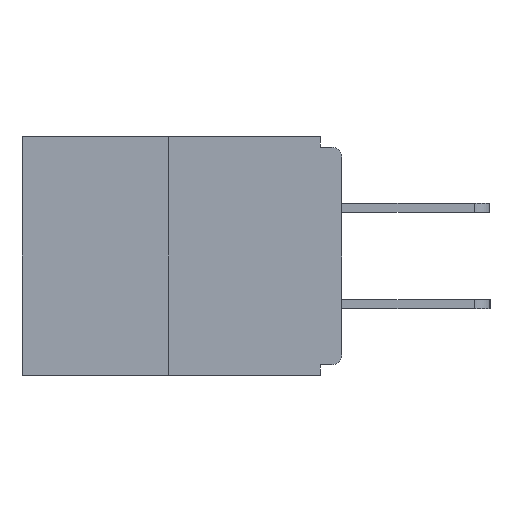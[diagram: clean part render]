
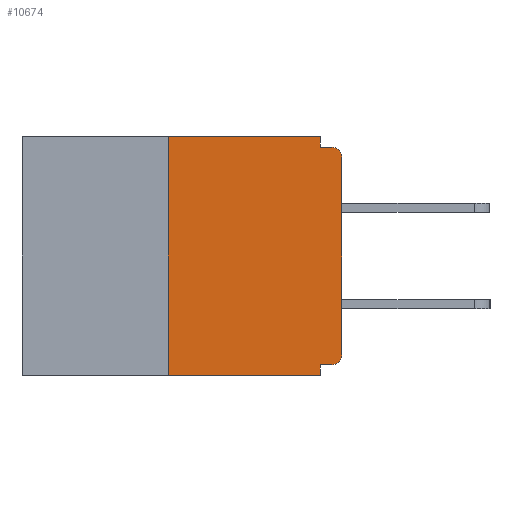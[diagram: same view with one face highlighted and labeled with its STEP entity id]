
A CAD part, left-side view. The second image highlights one B-rep face of the part: STEP entity #10674.
In plain terms, the highlighted planar face has unit normal (-1, 0, 0).
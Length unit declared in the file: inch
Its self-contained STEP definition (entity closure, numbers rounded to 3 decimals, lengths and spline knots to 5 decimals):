
#188 = LINE ( 'NONE', #837, #4559 ) ;
#520 = CARTESIAN_POINT ( 'NONE',  ( 0., 0.015, -0.03 ) ) ;
#718 = VECTOR ( 'NONE', #12293, 39.37008 ) ;
#837 = CARTESIAN_POINT ( 'NONE',  ( 0., 0., 0. ) ) ;
#1148 = VECTOR ( 'NONE', #7098, 39.37008 ) ;
#1250 = DIRECTION ( 'NONE',  ( 1., 0., 0. ) ) ;
#1312 = ORIENTED_EDGE ( 'NONE', *, *, #8876, .T. ) ;
#1439 = EDGE_LOOP ( 'NONE', ( #7261, #9956, #1312, #9376, #16176, #23420, #23938, #1974, #8960, #11372 ) ) ;
#1484 = CARTESIAN_POINT ( 'NONE',  ( 0., 0.031, -0.328 ) ) ;
#1597 = DIRECTION ( 'NONE',  ( 0., 0., 1. ) ) ;
#1974 = ORIENTED_EDGE ( 'NONE', *, *, #13596, .T. ) ;
#2115 = CARTESIAN_POINT ( 'NONE',  ( 0., 0., -0.313 ) ) ;
#2411 = LINE ( 'NONE', #10865, #6528 ) ;
#2457 = FACE_OUTER_BOUND ( 'NONE', #1439, .T. ) ;
#2822 = CARTESIAN_POINT ( 'NONE',  ( 0., 0., -0.015 ) ) ;
#3565 = EDGE_CURVE ( 'NONE', #16585, #7551, #13397, .T. ) ;
#3572 = CARTESIAN_POINT ( 'NONE',  ( 0., 0.46, -0.343 ) ) ;
#3648 = AXIS2_PLACEMENT_3D ( 'NONE', #520, #9982, #11940 ) ;
#4559 = VECTOR ( 'NONE', #19472, 39.37008 ) ;
#4700 = CARTESIAN_POINT ( 'NONE',  ( 0., 0.031, -0.015 ) ) ;
#4803 = CARTESIAN_POINT ( 'NONE',  ( 0., 0.46, 0. ) ) ;
#4838 = CARTESIAN_POINT ( 'NONE',  ( 0., 0.031, 0. ) ) ;
#5561 = LINE ( 'NONE', #3572, #15198 ) ;
#6234 = EDGE_CURVE ( 'NONE', #11658, #16585, #9492, .T. ) ;
#6528 = VECTOR ( 'NONE', #12492, 39.37008 ) ;
#7098 = DIRECTION ( 'NONE',  ( 0., -1., 0. ) ) ;
#7261 = ORIENTED_EDGE ( 'NONE', *, *, #6234, .F. ) ;
#7366 = DIRECTION ( 'NONE',  ( 0., -1., 0. ) ) ;
#7526 = CARTESIAN_POINT ( 'NONE',  ( 0., 0.25, 0. ) ) ;
#7551 = VERTEX_POINT ( 'NONE', #4700 ) ;
#7869 = VECTOR ( 'NONE', #9133, 39.37008 ) ;
#7979 = CARTESIAN_POINT ( 'NONE',  ( 0., 0.015, -0.313 ) ) ;
#8876 = EDGE_CURVE ( 'NONE', #20197, #20510, #5561, .T. ) ;
#8960 = ORIENTED_EDGE ( 'NONE', *, *, #22233, .F. ) ;
#9133 = DIRECTION ( 'NONE',  ( 0., 0., -1. ) ) ;
#9191 = CIRCLE ( 'NONE', #18291, 0.015 ) ;
#9376 = ORIENTED_EDGE ( 'NONE', *, *, #13749, .F. ) ;
#9492 = LINE ( 'NONE', #4803, #718 ) ;
#9520 = CARTESIAN_POINT ( 'NONE',  ( 0., 0.031, -0.343 ) ) ;
#9956 = ORIENTED_EDGE ( 'NONE', *, *, #10881, .F. ) ;
#9982 = DIRECTION ( 'NONE',  ( -1., 0., 0. ) ) ;
#10186 = CARTESIAN_POINT ( 'NONE',  ( 0., 0.015, -0.015 ) ) ;
#10621 = EDGE_CURVE ( 'NONE', #16329, #19788, #9191, .T. ) ;
#10674 = ADVANCED_FACE ( 'NONE', ( #2457 ), #16040, .F. ) ;
#10833 = CARTESIAN_POINT ( 'NONE',  ( 0., 0.25, -0.343 ) ) ;
#10856 = CARTESIAN_POINT ( 'NONE',  ( 0., 0.031, -0.343 ) ) ;
#10865 = CARTESIAN_POINT ( 'NONE',  ( 0., 0., -0.328 ) ) ;
#10881 = EDGE_CURVE ( 'NONE', #20197, #11658, #22971, .T. ) ;
#11372 = ORIENTED_EDGE ( 'NONE', *, *, #3565, .F. ) ;
#11658 = VERTEX_POINT ( 'NONE', #7526 ) ;
#11940 = DIRECTION ( 'NONE',  ( 0., 0., -1. ) ) ;
#12293 = DIRECTION ( 'NONE',  ( 0., -1., 0. ) ) ;
#12492 = DIRECTION ( 'NONE',  ( 0., 1., 0. ) ) ;
#12818 = VERTEX_POINT ( 'NONE', #10186 ) ;
#13397 = LINE ( 'NONE', #21056, #21026 ) ;
#13596 = EDGE_CURVE ( 'NONE', #20984, #12818, #18655, .T. ) ;
#13749 = EDGE_CURVE ( 'NONE', #21446, #20510, #22820, .T. ) ;
#14122 = VECTOR ( 'NONE', #1597, 39.37008 ) ;
#15198 = VECTOR ( 'NONE', #7366, 39.37008 ) ;
#16040 = PLANE ( 'NONE',  #16719 ) ;
#16176 = ORIENTED_EDGE ( 'NONE', *, *, #16833, .F. ) ;
#16329 = VERTEX_POINT ( 'NONE', #24001 ) ;
#16585 = VERTEX_POINT ( 'NONE', #4838 ) ;
#16719 = AXIS2_PLACEMENT_3D ( 'NONE', #23608, #1250, #19960 ) ;
#16833 = EDGE_CURVE ( 'NONE', #16329, #21446, #2411, .T. ) ;
#18291 = AXIS2_PLACEMENT_3D ( 'NONE', #7979, #21282, #21048 ) ;
#18655 = CIRCLE ( 'NONE', #3648, 0.015 ) ;
#19472 = DIRECTION ( 'NONE',  ( 0., 0., 1. ) ) ;
#19788 = VERTEX_POINT ( 'NONE', #2115 ) ;
#19960 = DIRECTION ( 'NONE',  ( 0., 0., -1. ) ) ;
#20197 = VERTEX_POINT ( 'NONE', #10833 ) ;
#20510 = VERTEX_POINT ( 'NONE', #9520 ) ;
#20531 = CARTESIAN_POINT ( 'NONE',  ( 0., 0., -0.03 ) ) ;
#20546 = EDGE_CURVE ( 'NONE', #19788, #20984, #188, .T. ) ;
#20984 = VERTEX_POINT ( 'NONE', #20531 ) ;
#21026 = VECTOR ( 'NONE', #22969, 39.37008 ) ;
#21048 = DIRECTION ( 'NONE',  ( 0., 0., -1. ) ) ;
#21056 = CARTESIAN_POINT ( 'NONE',  ( 0., 0.031, 0. ) ) ;
#21070 = LINE ( 'NONE', #2822, #1148 ) ;
#21282 = DIRECTION ( 'NONE',  ( -1., 0., 0. ) ) ;
#21446 = VERTEX_POINT ( 'NONE', #1484 ) ;
#22233 = EDGE_CURVE ( 'NONE', #7551, #12818, #21070, .T. ) ;
#22820 = LINE ( 'NONE', #10856, #7869 ) ;
#22969 = DIRECTION ( 'NONE',  ( 0., 0., -1. ) ) ;
#22971 = LINE ( 'NONE', #23778, #14122 ) ;
#23420 = ORIENTED_EDGE ( 'NONE', *, *, #10621, .T. ) ;
#23608 = CARTESIAN_POINT ( 'NONE',  ( 0., 0.46, 0. ) ) ;
#23778 = CARTESIAN_POINT ( 'NONE',  ( 0., 0.25, 0. ) ) ;
#23938 = ORIENTED_EDGE ( 'NONE', *, *, #20546, .T. ) ;
#24001 = CARTESIAN_POINT ( 'NONE',  ( 0., 0.015, -0.328 ) ) ;
